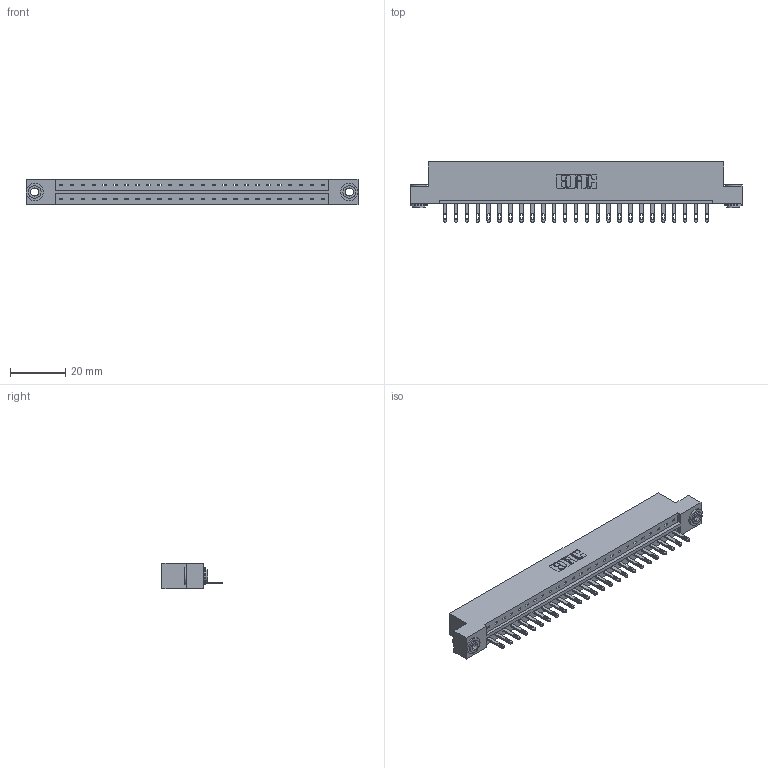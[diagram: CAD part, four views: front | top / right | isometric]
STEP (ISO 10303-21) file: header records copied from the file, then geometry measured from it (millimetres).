
FILE_DESCRIPTION (( 'STEP AP203' ), '1' );
FILE_NAME ('333-025-500-103.STEP', '2018-08-02T11:52:21', ( '' ), ( '' ), 'SwSTEP 2.0', 'SolidWorks 2016', '' );
FILE_SCHEMA (( 'CONFIG_CONTROL_DESIGN' ));
Length unit declared in the file: inch
Products named in the file (4): 333 Part_Flush - .156 Dia - TH; 345-292-001_345-293-100; 345-250-002_345-250-002-102; 333-025-500-103
Assembly tree (28 placements, depth 2):
  333-025-500-103
    333 Part_Flush - .156 Dia - TH
    345-292-001_345-293-100  x25
    345-250-002_345-250-002-102  x2
Bounding box: 120.6 x 21.85 x 9.4 mm (x, y, z)
Volume: 12024.3 mm3; surface area: 13187.2 mm2
Topology: 28 solids, 28 shells, 1502 faces, 4587 edges, 3054 vertices
Faces by surface type: plane 980, cylinder 514, cone 8
Entity records: 18062 total; most frequent: CARTESIAN_POINT 3096, ORIENTED_EDGE 3050, DIRECTION 2681, EDGE_CURVE 1525, LINE 1369, VECTOR 1369, VERTEX_POINT 1014, AXIS2_PLACEMENT_3D 656
